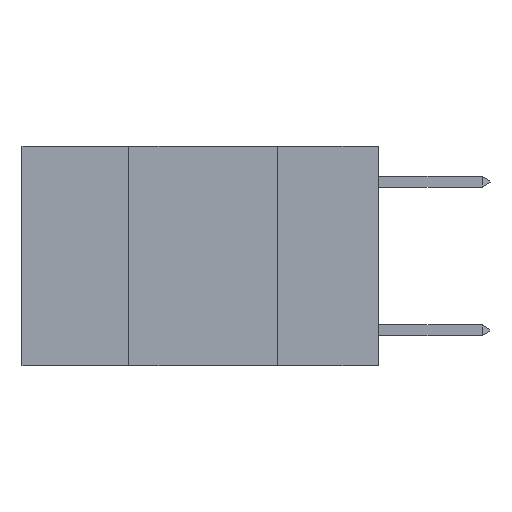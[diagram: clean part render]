
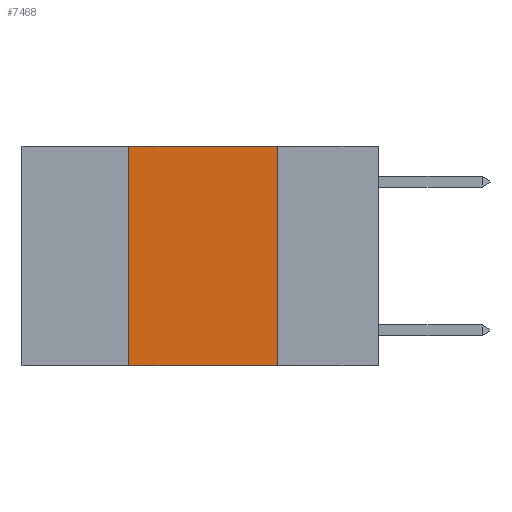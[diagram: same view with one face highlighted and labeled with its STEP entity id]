
A CAD part, left-side view. The second image highlights one B-rep face of the part: STEP entity #7468.
In plain terms, the highlighted planar face has unit normal (-1, 0, 0).
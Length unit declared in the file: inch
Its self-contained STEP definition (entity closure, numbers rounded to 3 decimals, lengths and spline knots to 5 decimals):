
#147 = DIRECTION ( 'NONE',  ( 1., 0., 0. ) ) ;
#284 = VECTOR ( 'NONE', #8778, 39.37008 ) ;
#546 = AXIS2_PLACEMENT_3D ( 'NONE', #5867, #147, #9104 ) ;
#582 = VERTEX_POINT ( 'NONE', #5950 ) ;
#1083 = ORIENTED_EDGE ( 'NONE', *, *, #6532, .F. ) ;
#1200 = DIRECTION ( 'NONE',  ( 0., -1., 0. ) ) ;
#1256 = CARTESIAN_POINT ( 'NONE',  ( 0., 0.6, -0.37 ) ) ;
#1516 = CARTESIAN_POINT ( 'NONE',  ( 0., 0.42, 0. ) ) ;
#1898 = LINE ( 'NONE', #1256, #10024 ) ;
#2378 = EDGE_LOOP ( 'NONE', ( #9606, #5073, #1083, #3633 ) ) ;
#2636 = FACE_OUTER_BOUND ( 'NONE', #2378, .T. ) ;
#2729 = CARTESIAN_POINT ( 'NONE',  ( 0., 0.42, -0.37 ) ) ;
#3633 = ORIENTED_EDGE ( 'NONE', *, *, #6349, .T. ) ;
#3730 = DIRECTION ( 'NONE',  ( 0., 0., 1. ) ) ;
#4420 = CARTESIAN_POINT ( 'NONE',  ( 0., 0.17, -0.37 ) ) ;
#4669 = EDGE_CURVE ( 'NONE', #4827, #582, #10128, .T. ) ;
#4753 = EDGE_CURVE ( 'NONE', #582, #8021, #5355, .T. ) ;
#4827 = VERTEX_POINT ( 'NONE', #7881 ) ;
#5073 = ORIENTED_EDGE ( 'NONE', *, *, #4669, .F. ) ;
#5355 = LINE ( 'NONE', #5402, #284 ) ;
#5402 = CARTESIAN_POINT ( 'NONE',  ( 0., 0.17, 0. ) ) ;
#5867 = CARTESIAN_POINT ( 'NONE',  ( 0., 0.6, 0. ) ) ;
#5950 = CARTESIAN_POINT ( 'NONE',  ( 0., 0.17, 0. ) ) ;
#6349 = EDGE_CURVE ( 'NONE', #6368, #8021, #1898, .T. ) ;
#6368 = VERTEX_POINT ( 'NONE', #2729 ) ;
#6532 = EDGE_CURVE ( 'NONE', #6368, #4827, #7131, .T. ) ;
#7131 = LINE ( 'NONE', #1516, #8321 ) ;
#7403 = PLANE ( 'NONE',  #546 ) ;
#7468 = ADVANCED_FACE ( 'NONE', ( #2636 ), #7403, .F. ) ;
#7573 = VECTOR ( 'NONE', #9914, 39.37008 ) ;
#7881 = CARTESIAN_POINT ( 'NONE',  ( 0., 0.42, 0. ) ) ;
#8021 = VERTEX_POINT ( 'NONE', #4420 ) ;
#8321 = VECTOR ( 'NONE', #3730, 39.37008 ) ;
#8778 = DIRECTION ( 'NONE',  ( 0., 0., -1. ) ) ;
#9104 = DIRECTION ( 'NONE',  ( 0., 0., -1. ) ) ;
#9314 = CARTESIAN_POINT ( 'NONE',  ( 0., 0.6, 0. ) ) ;
#9606 = ORIENTED_EDGE ( 'NONE', *, *, #4753, .F. ) ;
#9914 = DIRECTION ( 'NONE',  ( 0., -1., 0. ) ) ;
#10024 = VECTOR ( 'NONE', #1200, 39.37008 ) ;
#10128 = LINE ( 'NONE', #9314, #7573 ) ;
